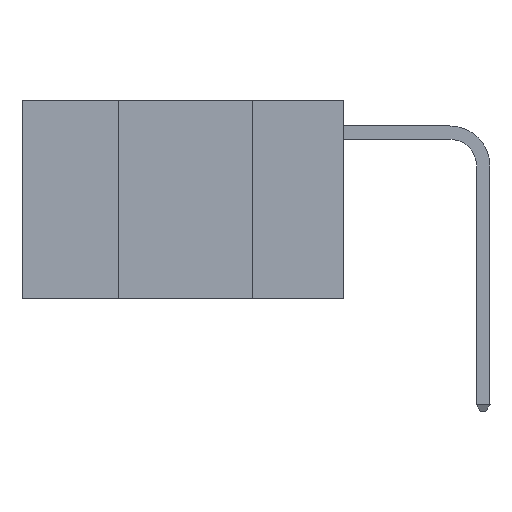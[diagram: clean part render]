
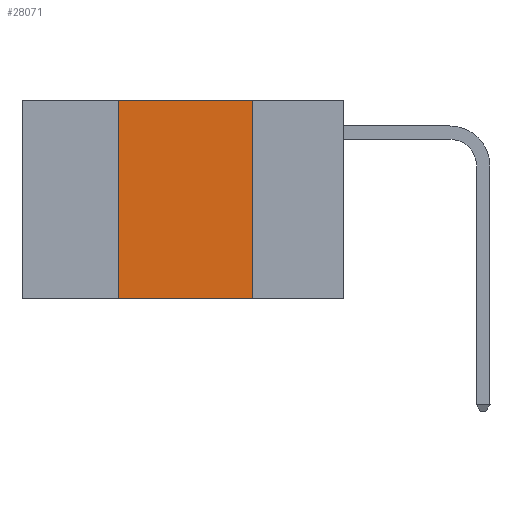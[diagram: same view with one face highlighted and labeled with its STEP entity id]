
A CAD part, left-side view. The second image highlights one B-rep face of the part: STEP entity #28071.
In plain terms, the highlighted planar face has unit normal (-1, 0, 0).
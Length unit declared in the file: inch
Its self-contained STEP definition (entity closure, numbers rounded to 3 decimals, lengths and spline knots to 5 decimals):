
#160 = CARTESIAN_POINT ( 'NONE',  ( 0., 0.17, 0. ) ) ;
#763 = EDGE_LOOP ( 'NONE', ( #17729, #19403, #29368, #22007 ) ) ;
#1285 = CARTESIAN_POINT ( 'NONE',  ( 0., 0.6, 0. ) ) ;
#2718 = VECTOR ( 'NONE', #6763, 39.37008 ) ;
#2764 = VERTEX_POINT ( 'NONE', #6179 ) ;
#3359 = DIRECTION ( 'NONE',  ( 0., -1., 0. ) ) ;
#3679 = FACE_OUTER_BOUND ( 'NONE', #763, .T. ) ;
#4139 = EDGE_CURVE ( 'NONE', #4588, #2764, #11307, .T. ) ;
#4588 = VERTEX_POINT ( 'NONE', #23764 ) ;
#4688 = LINE ( 'NONE', #9607, #2718 ) ;
#6179 = CARTESIAN_POINT ( 'NONE',  ( 0., 0.17, -0.37 ) ) ;
#6763 = DIRECTION ( 'NONE',  ( 0., 0., -1. ) ) ;
#7069 = EDGE_CURVE ( 'NONE', #31145, #2764, #4688, .T. ) ;
#9558 = DIRECTION ( 'NONE',  ( 1., 0., 0. ) ) ;
#9607 = CARTESIAN_POINT ( 'NONE',  ( 0., 0.17, 0. ) ) ;
#10298 = VECTOR ( 'NONE', #19525, 39.37008 ) ;
#11307 = LINE ( 'NONE', #18957, #10298 ) ;
#13091 = CARTESIAN_POINT ( 'NONE',  ( 0., 0.6, 0. ) ) ;
#13400 = PLANE ( 'NONE',  #16763 ) ;
#15558 = VECTOR ( 'NONE', #16384, 39.37008 ) ;
#16065 = LINE ( 'NONE', #23812, #15558 ) ;
#16384 = DIRECTION ( 'NONE',  ( 0., 0., 1. ) ) ;
#16573 = DIRECTION ( 'NONE',  ( 0., 0., -1. ) ) ;
#16763 = AXIS2_PLACEMENT_3D ( 'NONE', #1285, #9558, #16573 ) ;
#17729 = ORIENTED_EDGE ( 'NONE', *, *, #7069, .F. ) ;
#18957 = CARTESIAN_POINT ( 'NONE',  ( 0., 0.6, -0.37 ) ) ;
#19111 = VECTOR ( 'NONE', #3359, 39.37008 ) ;
#19403 = ORIENTED_EDGE ( 'NONE', *, *, #22065, .F. ) ;
#19525 = DIRECTION ( 'NONE',  ( 0., -1., 0. ) ) ;
#22007 = ORIENTED_EDGE ( 'NONE', *, *, #4139, .T. ) ;
#22065 = EDGE_CURVE ( 'NONE', #27296, #31145, #25105, .T. ) ;
#23764 = CARTESIAN_POINT ( 'NONE',  ( 0., 0.42, -0.37 ) ) ;
#23812 = CARTESIAN_POINT ( 'NONE',  ( 0., 0.42, 0. ) ) ;
#23814 = EDGE_CURVE ( 'NONE', #4588, #27296, #16065, .T. ) ;
#24998 = CARTESIAN_POINT ( 'NONE',  ( 0., 0.42, 0. ) ) ;
#25105 = LINE ( 'NONE', #13091, #19111 ) ;
#27296 = VERTEX_POINT ( 'NONE', #24998 ) ;
#28071 = ADVANCED_FACE ( 'NONE', ( #3679 ), #13400, .F. ) ;
#29368 = ORIENTED_EDGE ( 'NONE', *, *, #23814, .F. ) ;
#31145 = VERTEX_POINT ( 'NONE', #160 ) ;
